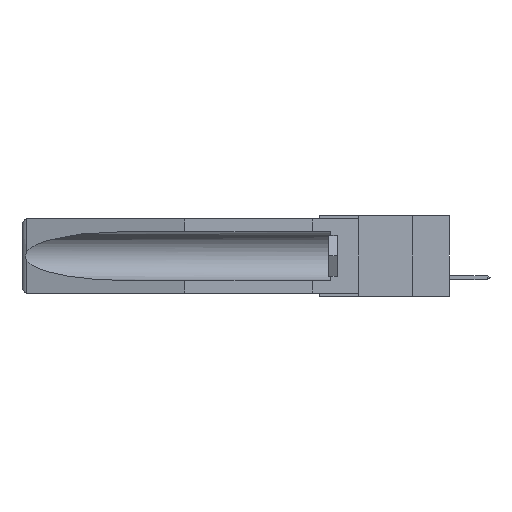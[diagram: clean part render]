
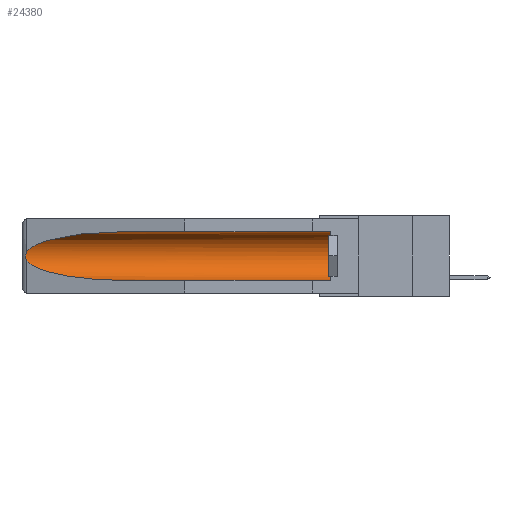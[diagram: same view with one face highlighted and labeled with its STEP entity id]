
A CAD part, left-side view. The second image highlights one B-rep face of the part: STEP entity #24380.
In plain terms, the highlighted cylindrical face has radius 2.857 mm (diameter 5.715 mm), a partial arc.
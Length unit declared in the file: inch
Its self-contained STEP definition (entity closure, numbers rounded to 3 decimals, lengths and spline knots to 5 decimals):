
#571 = CARTESIAN_POINT ( 'NONE',  ( 0.155, -0.30754, -0.284 ) ) ;
#620 = CARTESIAN_POINT ( 'NONE',  ( 0.2673, 1.5327, -0.16383 ) ) ;
#905 = CARTESIAN_POINT ( 'NONE',  ( 0.26655, 1.53094, -0.18657 ) ) ;
#1585 = CARTESIAN_POINT ( 'NONE',  ( 0.155, -0.30754, -0.059 ) ) ;
#2114 = VECTOR ( 'NONE', #3668, 39.37008 ) ;
#3668 = DIRECTION ( 'NONE',  ( 0., 1., 0. ) ) ;
#3685 = CARTESIAN_POINT ( 'NONE',  ( 0.155, 1.07973, -0.059 ) ) ;
#5386 = DIRECTION ( 'NONE',  ( 0., 0., 1. ) ) ;
#5735 = FACE_OUTER_BOUND ( 'NONE', #11347, .T. ) ;
#6408 = CARTESIAN_POINT ( 'NONE',  ( 0.21114, 1.30732, -0.284 ) ) ;
#7146 = VERTEX_POINT ( 'NONE', #15402 ) ;
#7561 = CARTESIAN_POINT ( 'NONE',  ( 0.155, 0.126, -0.1715 ) ) ;
#7704 = EDGE_CURVE ( 'NONE', #28002, #17961, #15344, .T. ) ;
#7770 = CARTESIAN_POINT ( 'NONE',  ( 0.155, 1.07973, -0.284 ) ) ;
#8142 =( BOUNDED_CURVE ( )  B_SPLINE_CURVE ( 3, ( #10169, #21280, #28488, #9972 ),
 .UNSPECIFIED., .F., .F. ) 
 B_SPLINE_CURVE_WITH_KNOTS ( ( 4, 4 ),
 ( 4.71239, 6.08839 ),
 .UNSPECIFIED. ) 
 CURVE ( )  GEOMETRIC_REPRESENTATION_ITEM ( )  RATIONAL_B_SPLINE_CURVE ( ( 1., 0.848, 0.848, 1. ) ) 
 REPRESENTATION_ITEM ( '' )  );
#8573 = CARTESIAN_POINT ( 'NONE',  ( 0.25451, 1.48313, -0.24835 ) ) ;
#9479 = EDGE_CURVE ( 'NONE', #7146, #28288, #24206, .T. ) ;
#9947 = CARTESIAN_POINT ( 'NONE',  ( 0.2675, 1.53308, -0.16763 ) ) ;
#9972 = CARTESIAN_POINT ( 'NONE',  ( 0.26537, 1.52718, -0.14972 ) ) ;
#10169 = CARTESIAN_POINT ( 'NONE',  ( 0.155, 1.07973, -0.059 ) ) ;
#11125 = CARTESIAN_POINT ( 'NONE',  ( 0.26537, 1.52718, -0.14972 ) ) ;
#11347 = EDGE_LOOP ( 'NONE', ( #24526, #13706, #23810, #16886, #25037, #28987 ) ) ;
#11554 = AXIS2_PLACEMENT_3D ( 'NONE', #23622, #26048, #14649 ) ;
#12156 = CARTESIAN_POINT ( 'NONE',  ( 0.26597, 1.5296, -0.19026 ) ) ;
#12254 = CARTESIAN_POINT ( 'NONE',  ( 0.2673, 1.53269, -0.17917 ) ) ;
#12977 = CARTESIAN_POINT ( 'NONE',  ( 0.26537, 1.52718, -0.19328 ) ) ;
#13706 = ORIENTED_EDGE ( 'NONE', *, *, #18456, .T. ) ;
#14235 = EDGE_CURVE ( 'NONE', #28002, #7146, #27450, .T. ) ;
#14280 = CARTESIAN_POINT ( 'NONE',  ( 0.26654, 1.53092, -0.15636 ) ) ;
#14294 = VERTEX_POINT ( 'NONE', #11125 ) ;
#14467 = CARTESIAN_POINT ( 'NONE',  ( 0.26537, 1.52718, -0.19328 ) ) ;
#14649 = DIRECTION ( 'NONE',  ( 0., 0., 1. ) ) ;
#15344 = LINE ( 'NONE', #571, #29366 ) ;
#15402 = CARTESIAN_POINT ( 'NONE',  ( 0.155, 0.126, -0.059 ) ) ;
#16749 = CARTESIAN_POINT ( 'NONE',  ( 0.26597, 1.52961, -0.15275 ) ) ;
#16886 = ORIENTED_EDGE ( 'NONE', *, *, #7704, .F. ) ;
#17961 = VERTEX_POINT ( 'NONE', #7770 ) ;
#17981 = CARTESIAN_POINT ( 'NONE',  ( 0.155, 0.126, -0.284 ) ) ;
#18456 = EDGE_CURVE ( 'NONE', #14294, #25300, #18780, .T. ) ;
#18780 = B_SPLINE_CURVE_WITH_KNOTS ( 'NONE', 3,
 ( #26160, #16749, #14280, #620, #9947, #25874, #12254, #905, #12156, #14467 ),
 .UNSPECIFIED., .F., .F.,
 ( 4, 2, 2, 2, 4 ),
 ( 0., 0.00029, 0.00058, 0.00087, 0.00117 ),
 .UNSPECIFIED. ) ;
#18930 = DIRECTION ( 'NONE',  ( 0., -1., 0. ) ) ;
#19115 = DIRECTION ( 'NONE',  ( 0., 1., 0. ) ) ;
#19142 = CARTESIAN_POINT ( 'NONE',  ( 0.26537, 1.52718, -0.19328 ) ) ;
#20929 = EDGE_CURVE ( 'NONE', #28288, #14294, #8142, .T. ) ;
#21280 = CARTESIAN_POINT ( 'NONE',  ( 0.21114, 1.30732, -0.059 ) ) ;
#21780 = CYLINDRICAL_SURFACE ( 'NONE', #11554, 0.1125 ) ;
#21877 =( BOUNDED_CURVE ( )  B_SPLINE_CURVE ( 3, ( #12977, #8573, #6408, #29198 ),
 .UNSPECIFIED., .F., .F. ) 
 B_SPLINE_CURVE_WITH_KNOTS ( ( 4, 4 ),
 ( 0.1948, 1.5708 ),
 .UNSPECIFIED. ) 
 CURVE ( )  GEOMETRIC_REPRESENTATION_ITEM ( )  RATIONAL_B_SPLINE_CURVE ( ( 1., 0.848, 0.848, 1. ) ) 
 REPRESENTATION_ITEM ( '' )  );
#22970 = EDGE_CURVE ( 'NONE', #25300, #17961, #21877, .T. ) ;
#23622 = CARTESIAN_POINT ( 'NONE',  ( 0.155, -0.30754, -0.1715 ) ) ;
#23810 = ORIENTED_EDGE ( 'NONE', *, *, #22970, .T. ) ;
#24206 = LINE ( 'NONE', #1585, #2114 ) ;
#24380 = ADVANCED_FACE ( 'NONE', ( #5735 ), #21780, .F. ) ;
#24526 = ORIENTED_EDGE ( 'NONE', *, *, #20929, .T. ) ;
#25037 = ORIENTED_EDGE ( 'NONE', *, *, #14235, .T. ) ;
#25300 = VERTEX_POINT ( 'NONE', #19142 ) ;
#25350 = AXIS2_PLACEMENT_3D ( 'NONE', #7561, #18930, #5386 ) ;
#25874 = CARTESIAN_POINT ( 'NONE',  ( 0.2675, 1.53308, -0.17534 ) ) ;
#26048 = DIRECTION ( 'NONE',  ( 0., 1., 0. ) ) ;
#26160 = CARTESIAN_POINT ( 'NONE',  ( 0.26537, 1.52718, -0.14972 ) ) ;
#27450 = CIRCLE ( 'NONE', #25350, 0.1125 ) ;
#28002 = VERTEX_POINT ( 'NONE', #17981 ) ;
#28288 = VERTEX_POINT ( 'NONE', #3685 ) ;
#28488 = CARTESIAN_POINT ( 'NONE',  ( 0.25451, 1.48313, -0.09465 ) ) ;
#28987 = ORIENTED_EDGE ( 'NONE', *, *, #9479, .T. ) ;
#29198 = CARTESIAN_POINT ( 'NONE',  ( 0.155, 1.07973, -0.284 ) ) ;
#29366 = VECTOR ( 'NONE', #19115, 39.37008 ) ;
